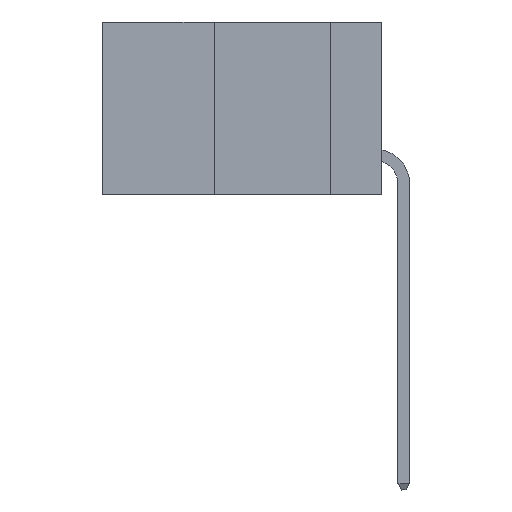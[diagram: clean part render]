
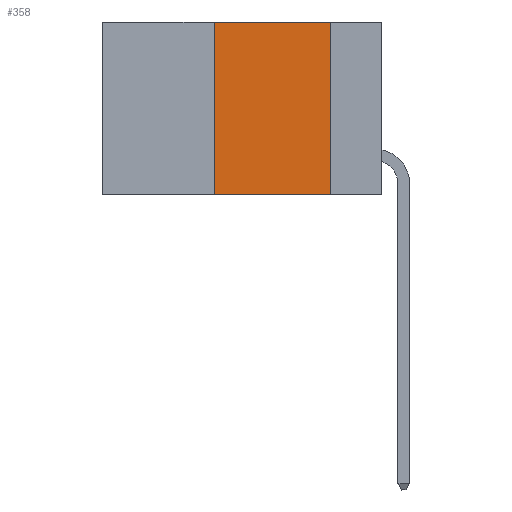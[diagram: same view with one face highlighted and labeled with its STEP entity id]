
A CAD part, left-side view. The second image highlights one B-rep face of the part: STEP entity #358.
In plain terms, the highlighted planar face has unit normal (-1, 0, 0).
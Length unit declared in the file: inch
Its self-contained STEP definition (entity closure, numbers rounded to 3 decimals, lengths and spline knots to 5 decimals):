
#358 = ADVANCED_FACE ( 'NONE', ( #8256 ), #4586, .F. ) ;
#1099 = CARTESIAN_POINT ( 'NONE',  ( 0., 0.11, 0. ) ) ;
#1885 = CARTESIAN_POINT ( 'NONE',  ( 0., 0.36, -0.37 ) ) ;
#3042 = AXIS2_PLACEMENT_3D ( 'NONE', #10639, #12012, #4670 ) ;
#3165 = LINE ( 'NONE', #16721, #13286 ) ;
#3577 = EDGE_CURVE ( 'NONE', #10269, #17179, #3165, .T. ) ;
#4089 = ORIENTED_EDGE ( 'NONE', *, *, #18755, .T. ) ;
#4586 = PLANE ( 'NONE',  #3042 ) ;
#4670 = DIRECTION ( 'NONE',  ( 0., 0., -1. ) ) ;
#4672 = EDGE_CURVE ( 'NONE', #17179, #16202, #13944, .T. ) ;
#6540 = CARTESIAN_POINT ( 'NONE',  ( 0., 0.6, 0. ) ) ;
#6656 = VECTOR ( 'NONE', #16078, 39.37008 ) ;
#7768 = VERTEX_POINT ( 'NONE', #8906 ) ;
#8256 = FACE_OUTER_BOUND ( 'NONE', #18151, .T. ) ;
#8906 = CARTESIAN_POINT ( 'NONE',  ( 0., 0.11, -0.37 ) ) ;
#9234 = LINE ( 'NONE', #16264, #6656 ) ;
#10269 = VERTEX_POINT ( 'NONE', #1885 ) ;
#10639 = CARTESIAN_POINT ( 'NONE',  ( 0., 0.6, 0. ) ) ;
#11408 = ORIENTED_EDGE ( 'NONE', *, *, #3577, .F. ) ;
#12011 = LINE ( 'NONE', #17821, #12481 ) ;
#12012 = DIRECTION ( 'NONE',  ( 1., 0., 0. ) ) ;
#12481 = VECTOR ( 'NONE', #16242, 39.37008 ) ;
#13286 = VECTOR ( 'NONE', #18376, 39.37008 ) ;
#13944 = LINE ( 'NONE', #6540, #16950 ) ;
#14576 = ORIENTED_EDGE ( 'NONE', *, *, #4672, .F. ) ;
#14661 = CARTESIAN_POINT ( 'NONE',  ( 0., 0.36, 0. ) ) ;
#15530 = ORIENTED_EDGE ( 'NONE', *, *, #16565, .F. ) ;
#16078 = DIRECTION ( 'NONE',  ( 0., -1., 0. ) ) ;
#16202 = VERTEX_POINT ( 'NONE', #1099 ) ;
#16242 = DIRECTION ( 'NONE',  ( 0., 0., -1. ) ) ;
#16264 = CARTESIAN_POINT ( 'NONE',  ( 0., 0.6, -0.37 ) ) ;
#16565 = EDGE_CURVE ( 'NONE', #16202, #7768, #12011, .T. ) ;
#16721 = CARTESIAN_POINT ( 'NONE',  ( 0., 0.36, 0. ) ) ;
#16950 = VECTOR ( 'NONE', #18361, 39.37008 ) ;
#17179 = VERTEX_POINT ( 'NONE', #14661 ) ;
#17821 = CARTESIAN_POINT ( 'NONE',  ( 0., 0.11, 0. ) ) ;
#18151 = EDGE_LOOP ( 'NONE', ( #15530, #14576, #11408, #4089 ) ) ;
#18361 = DIRECTION ( 'NONE',  ( 0., -1., 0. ) ) ;
#18376 = DIRECTION ( 'NONE',  ( 0., 0., 1. ) ) ;
#18755 = EDGE_CURVE ( 'NONE', #10269, #7768, #9234, .T. ) ;
